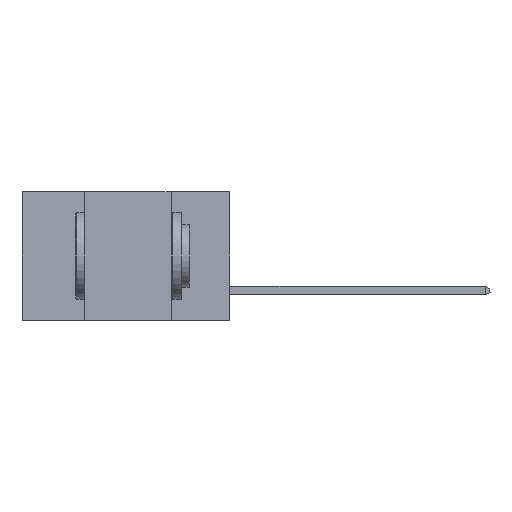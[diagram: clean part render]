
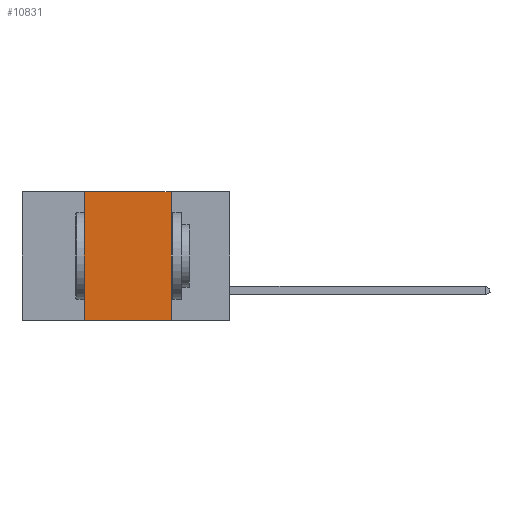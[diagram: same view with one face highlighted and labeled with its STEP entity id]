
A CAD part, left-side view. The second image highlights one B-rep face of the part: STEP entity #10831.
In plain terms, the highlighted planar face has unit normal (-1, 0, 0).
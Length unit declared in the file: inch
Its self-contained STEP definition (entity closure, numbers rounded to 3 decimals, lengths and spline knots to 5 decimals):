
#8 = VERTEX_POINT ( 'NONE', #9369 ) ;
#180 = CARTESIAN_POINT ( 'NONE',  ( 0., 0.6, 0. ) ) ;
#686 = LINE ( 'NONE', #17545, #18513 ) ;
#828 = VERTEX_POINT ( 'NONE', #14331 ) ;
#2152 = ORIENTED_EDGE ( 'NONE', *, *, #26893, .F. ) ;
#2622 = DIRECTION ( 'NONE',  ( 0., 0., -1. ) ) ;
#3624 = VECTOR ( 'NONE', #9184, 39.37008 ) ;
#7630 = EDGE_CURVE ( 'NONE', #8, #828, #29107, .T. ) ;
#9184 = DIRECTION ( 'NONE',  ( 0., -1., 0. ) ) ;
#9369 = CARTESIAN_POINT ( 'NONE',  ( 0., 0.42, -0.37 ) ) ;
#9798 = LINE ( 'NONE', #13734, #3624 ) ;
#10425 = CARTESIAN_POINT ( 'NONE',  ( 0., 0.17, 0. ) ) ;
#10633 = DIRECTION ( 'NONE',  ( 0., -1., 0. ) ) ;
#10831 = ADVANCED_FACE ( 'NONE', ( #25422 ), #23361, .F. ) ;
#10880 = CARTESIAN_POINT ( 'NONE',  ( 0., 0.17, -0.37 ) ) ;
#11366 = LINE ( 'NONE', #10425, #16748 ) ;
#11816 = EDGE_LOOP ( 'NONE', ( #19156, #2152, #17354, #24237 ) ) ;
#12443 = VERTEX_POINT ( 'NONE', #27063 ) ;
#13720 = VERTEX_POINT ( 'NONE', #10880 ) ;
#13734 = CARTESIAN_POINT ( 'NONE',  ( 0., 0.6, -0.37 ) ) ;
#14331 = CARTESIAN_POINT ( 'NONE',  ( 0., 0.42, 0. ) ) ;
#14921 = AXIS2_PLACEMENT_3D ( 'NONE', #180, #16486, #2622 ) ;
#15570 = DIRECTION ( 'NONE',  ( 0., 0., 1. ) ) ;
#16486 = DIRECTION ( 'NONE',  ( 1., 0., 0. ) ) ;
#16748 = VECTOR ( 'NONE', #28801, 39.37008 ) ;
#17354 = ORIENTED_EDGE ( 'NONE', *, *, #7630, .F. ) ;
#17545 = CARTESIAN_POINT ( 'NONE',  ( 0., 0.6, 0. ) ) ;
#18513 = VECTOR ( 'NONE', #10633, 39.37008 ) ;
#19156 = ORIENTED_EDGE ( 'NONE', *, *, #20126, .F. ) ;
#20126 = EDGE_CURVE ( 'NONE', #12443, #13720, #11366, .T. ) ;
#20214 = CARTESIAN_POINT ( 'NONE',  ( 0., 0.42, 0. ) ) ;
#21872 = EDGE_CURVE ( 'NONE', #8, #13720, #9798, .T. ) ;
#23361 = PLANE ( 'NONE',  #14921 ) ;
#24237 = ORIENTED_EDGE ( 'NONE', *, *, #21872, .T. ) ;
#25422 = FACE_OUTER_BOUND ( 'NONE', #11816, .T. ) ;
#26288 = VECTOR ( 'NONE', #15570, 39.37008 ) ;
#26893 = EDGE_CURVE ( 'NONE', #828, #12443, #686, .T. ) ;
#27063 = CARTESIAN_POINT ( 'NONE',  ( 0., 0.17, 0. ) ) ;
#28801 = DIRECTION ( 'NONE',  ( 0., 0., -1. ) ) ;
#29107 = LINE ( 'NONE', #20214, #26288 ) ;
